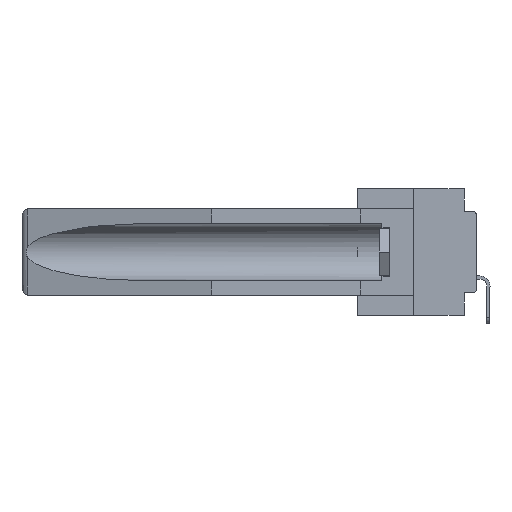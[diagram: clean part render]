
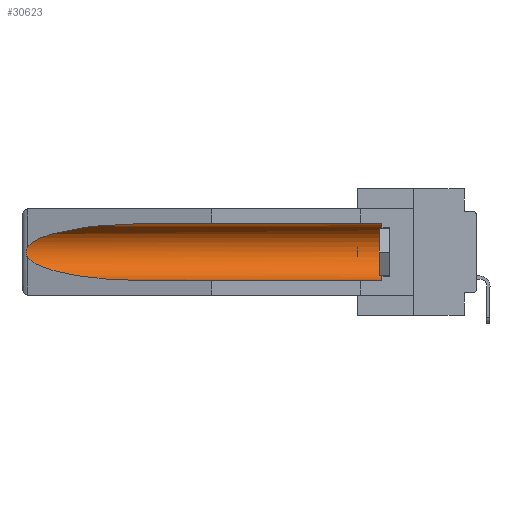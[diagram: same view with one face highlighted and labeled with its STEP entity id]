
A CAD part, left-side view. The second image highlights one B-rep face of the part: STEP entity #30623.
In plain terms, the highlighted cylindrical face has radius 2.857 mm (diameter 5.715 mm), a partial arc.
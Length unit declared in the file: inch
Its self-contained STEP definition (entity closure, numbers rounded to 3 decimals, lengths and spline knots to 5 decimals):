
#171 = CARTESIAN_POINT ( 'NONE',  ( 0.25451, 1.48313, -0.09465 ) ) ;
#590 = DIRECTION ( 'NONE',  ( 0., 0., 1. ) ) ;
#795 = ORIENTED_EDGE ( 'NONE', *, *, #11543, .T. ) ;
#1361 = DIRECTION ( 'NONE',  ( 0., -1., 0. ) ) ;
#1634 = CARTESIAN_POINT ( 'NONE',  ( 0.2673, 1.5327, -0.16383 ) ) ;
#3638 = VERTEX_POINT ( 'NONE', #23895 ) ;
#3788 = CARTESIAN_POINT ( 'NONE',  ( 0.155, 1.07973, -0.059 ) ) ;
#4556 = LINE ( 'NONE', #27474, #26634 ) ;
#4614 = EDGE_CURVE ( 'NONE', #10276, #40053, #11562, .T. ) ;
#4681 = CARTESIAN_POINT ( 'NONE',  ( 0.2675, 1.53308, -0.16763 ) ) ;
#5943 = ORIENTED_EDGE ( 'NONE', *, *, #4614, .T. ) ;
#6197 = DIRECTION ( 'NONE',  ( 0., 1., 0. ) ) ;
#7688 = CARTESIAN_POINT ( 'NONE',  ( 0.26537, 1.52718, -0.19328 ) ) ;
#7737 = ORIENTED_EDGE ( 'NONE', *, *, #36767, .T. ) ;
#9770 = B_SPLINE_CURVE_WITH_KNOTS ( 'NONE', 3,
 ( #17010, #29935, #17288, #1634, #4681, #26756, #26353, #39024, #10678, #7688 ),
 .UNSPECIFIED., .F., .F.,
 ( 4, 2, 2, 2, 4 ),
 ( 0., 0.00029, 0.00058, 0.00087, 0.00117 ),
 .UNSPECIFIED. ) ;
#10276 = VERTEX_POINT ( 'NONE', #3788 ) ;
#10678 = CARTESIAN_POINT ( 'NONE',  ( 0.26597, 1.5296, -0.19026 ) ) ;
#10696 = AXIS2_PLACEMENT_3D ( 'NONE', #16653, #26007, #590 ) ;
#11242 = CYLINDRICAL_SURFACE ( 'NONE', #10696, 0.1125 ) ;
#11543 = EDGE_CURVE ( 'NONE', #40053, #17731, #9770, .T. ) ;
#11562 =( BOUNDED_CURVE ( )  B_SPLINE_CURVE ( 3, ( #38125, #34809, #171, #13087 ),
 .UNSPECIFIED., .F., .F. ) 
 B_SPLINE_CURVE_WITH_KNOTS ( ( 4, 4 ),
 ( 4.71239, 6.08839 ),
 .UNSPECIFIED. ) 
 CURVE ( )  GEOMETRIC_REPRESENTATION_ITEM ( )  RATIONAL_B_SPLINE_CURVE ( ( 1., 0.848, 0.848, 1. ) ) 
 REPRESENTATION_ITEM ( '' )  );
#13087 = CARTESIAN_POINT ( 'NONE',  ( 0.26537, 1.52718, -0.14972 ) ) ;
#13619 = CARTESIAN_POINT ( 'NONE',  ( 0.25451, 1.48313, -0.24835 ) ) ;
#13865 = DIRECTION ( 'NONE',  ( 0., 0., 1. ) ) ;
#16530 = LINE ( 'NONE', #22211, #22441 ) ;
#16653 = CARTESIAN_POINT ( 'NONE',  ( 0.155, -0.30754, -0.1715 ) ) ;
#17010 = CARTESIAN_POINT ( 'NONE',  ( 0.26537, 1.52718, -0.14972 ) ) ;
#17021 = CARTESIAN_POINT ( 'NONE',  ( 0.155, 0.126, -0.1715 ) ) ;
#17288 = CARTESIAN_POINT ( 'NONE',  ( 0.26654, 1.53092, -0.15636 ) ) ;
#17731 = VERTEX_POINT ( 'NONE', #35514 ) ;
#18772 = EDGE_CURVE ( 'NONE', #3638, #38945, #16530, .T. ) ;
#19659 = ORIENTED_EDGE ( 'NONE', *, *, #31288, .T. ) ;
#21887 = EDGE_CURVE ( 'NONE', #17731, #38945, #25149, .T. ) ;
#22211 = CARTESIAN_POINT ( 'NONE',  ( 0.155, -0.30754, -0.284 ) ) ;
#22441 = VECTOR ( 'NONE', #28252, 39.37008 ) ;
#23895 = CARTESIAN_POINT ( 'NONE',  ( 0.155, 0.126, -0.284 ) ) ;
#24516 = FACE_OUTER_BOUND ( 'NONE', #37721, .T. ) ;
#24883 = ORIENTED_EDGE ( 'NONE', *, *, #21887, .T. ) ;
#25149 =( BOUNDED_CURVE ( )  B_SPLINE_CURVE ( 3, ( #29269, #13619, #26385, #39060 ),
 .UNSPECIFIED., .F., .F. ) 
 B_SPLINE_CURVE_WITH_KNOTS ( ( 4, 4 ),
 ( 0.1948, 1.5708 ),
 .UNSPECIFIED. ) 
 CURVE ( )  GEOMETRIC_REPRESENTATION_ITEM ( )  RATIONAL_B_SPLINE_CURVE ( ( 1., 0.848, 0.848, 1. ) ) 
 REPRESENTATION_ITEM ( '' )  );
#26007 = DIRECTION ( 'NONE',  ( 0., 1., 0. ) ) ;
#26086 = CARTESIAN_POINT ( 'NONE',  ( 0.26537, 1.52718, -0.14972 ) ) ;
#26353 = CARTESIAN_POINT ( 'NONE',  ( 0.2673, 1.53269, -0.17917 ) ) ;
#26385 = CARTESIAN_POINT ( 'NONE',  ( 0.21114, 1.30732, -0.284 ) ) ;
#26634 = VECTOR ( 'NONE', #6197, 39.37008 ) ;
#26756 = CARTESIAN_POINT ( 'NONE',  ( 0.2675, 1.53308, -0.17534 ) ) ;
#27474 = CARTESIAN_POINT ( 'NONE',  ( 0.155, -0.30754, -0.059 ) ) ;
#28252 = DIRECTION ( 'NONE',  ( 0., 1., 0. ) ) ;
#28374 = CIRCLE ( 'NONE', #32075, 0.1125 ) ;
#29269 = CARTESIAN_POINT ( 'NONE',  ( 0.26537, 1.52718, -0.19328 ) ) ;
#29935 = CARTESIAN_POINT ( 'NONE',  ( 0.26597, 1.52961, -0.15275 ) ) ;
#30623 = ADVANCED_FACE ( 'NONE', ( #24516 ), #11242, .F. ) ;
#31009 = CARTESIAN_POINT ( 'NONE',  ( 0.155, 0.126, -0.059 ) ) ;
#31288 = EDGE_CURVE ( 'NONE', #3638, #40574, #28374, .T. ) ;
#32075 = AXIS2_PLACEMENT_3D ( 'NONE', #17021, #1361, #13865 ) ;
#33603 = CARTESIAN_POINT ( 'NONE',  ( 0.155, 1.07973, -0.284 ) ) ;
#34809 = CARTESIAN_POINT ( 'NONE',  ( 0.21114, 1.30732, -0.059 ) ) ;
#35514 = CARTESIAN_POINT ( 'NONE',  ( 0.26537, 1.52718, -0.19328 ) ) ;
#36767 = EDGE_CURVE ( 'NONE', #40574, #10276, #4556, .T. ) ;
#37018 = ORIENTED_EDGE ( 'NONE', *, *, #18772, .F. ) ;
#37721 = EDGE_LOOP ( 'NONE', ( #5943, #795, #24883, #37018, #19659, #7737 ) ) ;
#38125 = CARTESIAN_POINT ( 'NONE',  ( 0.155, 1.07973, -0.059 ) ) ;
#38945 = VERTEX_POINT ( 'NONE', #33603 ) ;
#39024 = CARTESIAN_POINT ( 'NONE',  ( 0.26655, 1.53094, -0.18657 ) ) ;
#39060 = CARTESIAN_POINT ( 'NONE',  ( 0.155, 1.07973, -0.284 ) ) ;
#40053 = VERTEX_POINT ( 'NONE', #26086 ) ;
#40574 = VERTEX_POINT ( 'NONE', #31009 ) ;
